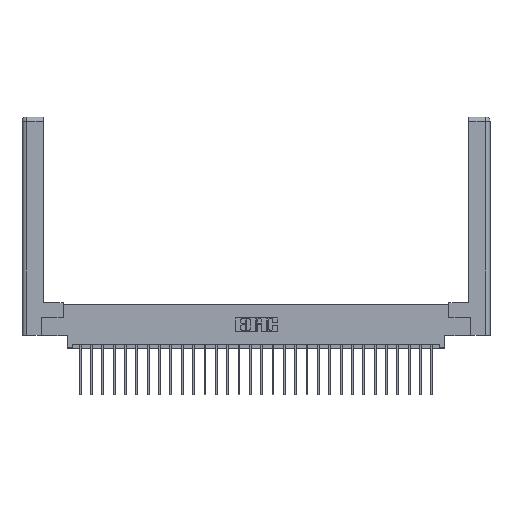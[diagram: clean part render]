
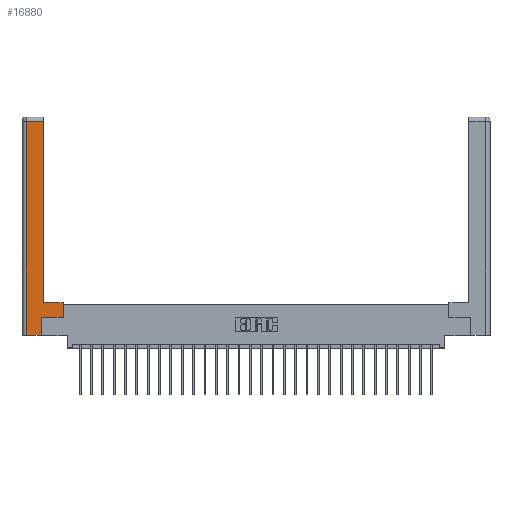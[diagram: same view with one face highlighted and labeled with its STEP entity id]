
A CAD part, top view. The second image highlights one B-rep face of the part: STEP entity #16880.
In plain terms, the highlighted planar face has unit normal (0, 0, 1).
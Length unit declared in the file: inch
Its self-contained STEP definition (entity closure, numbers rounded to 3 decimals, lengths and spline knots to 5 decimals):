
#189 = VECTOR ( 'NONE', #24590, 39.37008 ) ;
#204 = VECTOR ( 'NONE', #11624, 39.37008 ) ;
#1220 = EDGE_LOOP ( 'NONE', ( #12538, #5556, #12472, #25430, #13743, #23809, #22508, #22493 ) ) ;
#1983 = LINE ( 'NONE', #25012, #204 ) ;
#2169 = DIRECTION ( 'NONE',  ( 0., -1., 0. ) ) ;
#2936 = LINE ( 'NONE', #18936, #15542 ) ;
#3190 = CARTESIAN_POINT ( 'NONE',  ( 0.565, 0.245, 0. ) ) ;
#3604 = LINE ( 'NONE', #17500, #6075 ) ;
#5184 = CARTESIAN_POINT ( 'NONE',  ( 0.295, 0.45, 0. ) ) ;
#5556 = ORIENTED_EDGE ( 'NONE', *, *, #13096, .T. ) ;
#5557 = VERTEX_POINT ( 'NONE', #22730 ) ;
#6025 = LINE ( 'NONE', #14636, #14362 ) ;
#6075 = VECTOR ( 'NONE', #15551, 39.37008 ) ;
#6181 = AXIS2_PLACEMENT_3D ( 'NONE', #7593, #23193, #12463 ) ;
#6393 = LINE ( 'NONE', #28791, #7434 ) ;
#6582 = EDGE_CURVE ( 'NONE', #6655, #10959, #3604, .T. ) ;
#6655 = VERTEX_POINT ( 'NONE', #15647 ) ;
#7242 = DIRECTION ( 'NONE',  ( -1., 0., 0. ) ) ;
#7434 = VECTOR ( 'NONE', #2169, 39.37008 ) ;
#7593 = CARTESIAN_POINT ( 'NONE',  ( 0., 0., 0. ) ) ;
#7940 = CARTESIAN_POINT ( 'NONE',  ( 0.565, 0.45, 0. ) ) ;
#8322 = LINE ( 'NONE', #13913, #11309 ) ;
#8745 = VERTEX_POINT ( 'NONE', #3190 ) ;
#8986 = EDGE_CURVE ( 'NONE', #8745, #19935, #1983, .T. ) ;
#10704 = EDGE_CURVE ( 'NONE', #19935, #18416, #16229, .T. ) ;
#10959 = VERTEX_POINT ( 'NONE', #17970 ) ;
#11309 = VECTOR ( 'NONE', #15984, 39.37008 ) ;
#11624 = DIRECTION ( 'NONE',  ( 0., 1., 0. ) ) ;
#12106 = DIRECTION ( 'NONE',  ( 1., 0., 0. ) ) ;
#12463 = DIRECTION ( 'NONE',  ( -1., 0., 0. ) ) ;
#12472 = ORIENTED_EDGE ( 'NONE', *, *, #15846, .T. ) ;
#12538 = ORIENTED_EDGE ( 'NONE', *, *, #18982, .T. ) ;
#13096 = EDGE_CURVE ( 'NONE', #21494, #27356, #2936, .T. ) ;
#13743 = ORIENTED_EDGE ( 'NONE', *, *, #6582, .T. ) ;
#13811 = CARTESIAN_POINT ( 'NONE',  ( 0.295, 3., 0. ) ) ;
#13913 = CARTESIAN_POINT ( 'NONE',  ( 0.565, 0.245, 0. ) ) ;
#14362 = VECTOR ( 'NONE', #12106, 39.37008 ) ;
#14636 = CARTESIAN_POINT ( 'NONE',  ( 0.265, 0., 0. ) ) ;
#14842 = VECTOR ( 'NONE', #7242, 39.37008 ) ;
#15542 = VECTOR ( 'NONE', #18841, 39.37008 ) ;
#15551 = DIRECTION ( 'NONE',  ( 0., 1., 0. ) ) ;
#15647 = CARTESIAN_POINT ( 'NONE',  ( 0.265, 0., 0. ) ) ;
#15846 = EDGE_CURVE ( 'NONE', #27356, #5557, #6393, .T. ) ;
#15984 = DIRECTION ( 'NONE',  ( 1., 0., 0. ) ) ;
#16079 = FACE_OUTER_BOUND ( 'NONE', #1220, .T. ) ;
#16169 = EDGE_CURVE ( 'NONE', #5557, #6655, #6025, .T. ) ;
#16198 = CARTESIAN_POINT ( 'NONE',  ( 0.295, 0.45, 0. ) ) ;
#16229 = LINE ( 'NONE', #16198, #14842 ) ;
#16880 = ADVANCED_FACE ( 'NONE', ( #16079 ), #20927, .F. ) ;
#17500 = CARTESIAN_POINT ( 'NONE',  ( 0.265, 0.245, 0. ) ) ;
#17970 = CARTESIAN_POINT ( 'NONE',  ( 0.265, 0.245, 0. ) ) ;
#18416 = VERTEX_POINT ( 'NONE', #5184 ) ;
#18841 = DIRECTION ( 'NONE',  ( -1., 0., 0. ) ) ;
#18936 = CARTESIAN_POINT ( 'NONE',  ( 0.0615, 2.94, 0. ) ) ;
#18982 = EDGE_CURVE ( 'NONE', #18416, #21494, #24993, .T. ) ;
#19935 = VERTEX_POINT ( 'NONE', #7940 ) ;
#20923 = EDGE_CURVE ( 'NONE', #10959, #8745, #8322, .T. ) ;
#20927 = PLANE ( 'NONE',  #6181 ) ;
#21494 = VERTEX_POINT ( 'NONE', #26777 ) ;
#22493 = ORIENTED_EDGE ( 'NONE', *, *, #10704, .T. ) ;
#22508 = ORIENTED_EDGE ( 'NONE', *, *, #8986, .T. ) ;
#22730 = CARTESIAN_POINT ( 'NONE',  ( 0.0615, 0., 0. ) ) ;
#23193 = DIRECTION ( 'NONE',  ( 0., 0., -1. ) ) ;
#23809 = ORIENTED_EDGE ( 'NONE', *, *, #20923, .T. ) ;
#24448 = CARTESIAN_POINT ( 'NONE',  ( 0.0615, 2.94, 0. ) ) ;
#24590 = DIRECTION ( 'NONE',  ( 0., 1., 0. ) ) ;
#24993 = LINE ( 'NONE', #13811, #189 ) ;
#25012 = CARTESIAN_POINT ( 'NONE',  ( 0.565, 0.45, 0. ) ) ;
#25430 = ORIENTED_EDGE ( 'NONE', *, *, #16169, .T. ) ;
#26777 = CARTESIAN_POINT ( 'NONE',  ( 0.295, 2.94, 0. ) ) ;
#27356 = VERTEX_POINT ( 'NONE', #24448 ) ;
#28791 = CARTESIAN_POINT ( 'NONE',  ( 0.0615, 0., 0. ) ) ;
